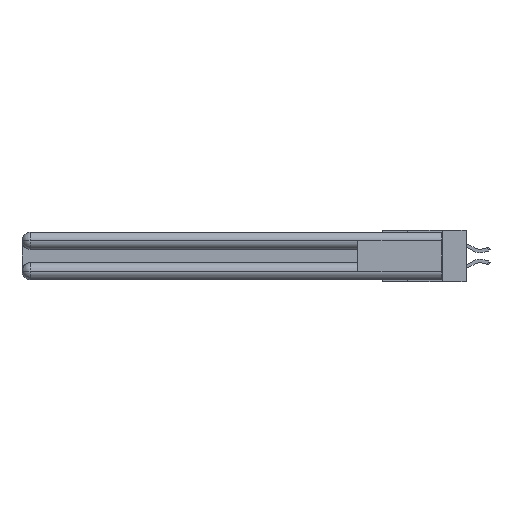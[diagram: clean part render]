
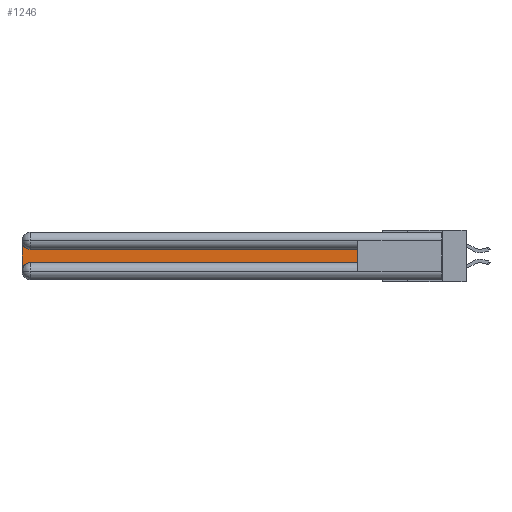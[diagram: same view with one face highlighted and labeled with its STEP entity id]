
A CAD part, left-side view. The second image highlights one B-rep face of the part: STEP entity #1246.
In plain terms, the highlighted planar face has unit normal (-1, 0, 0).
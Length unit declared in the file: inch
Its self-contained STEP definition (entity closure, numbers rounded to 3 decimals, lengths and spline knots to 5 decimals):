
#1246 = ADVANCED_FACE ( 'NONE', ( #10459 ), #15088, .F. ) ;
#3960 = AXIS2_PLACEMENT_3D ( 'NONE', #13023, #15390, #19690 ) ;
#4750 = CARTESIAN_POINT ( 'NONE',  ( 0.075, 3., -0.0625 ) ) ;
#5403 = DIRECTION ( 'NONE',  ( 0., 1., 0. ) ) ;
#7735 = DIRECTION ( 'NONE',  ( 1., 0., 0. ) ) ;
#7924 = AXIS2_PLACEMENT_3D ( 'NONE', #18759, #21262, #21171 ) ;
#8224 = ORIENTED_EDGE ( 'NONE', *, *, #29377, .T. ) ;
#9787 = DIRECTION ( 'NONE',  ( 0., 0., 1. ) ) ;
#9910 = CARTESIAN_POINT ( 'NONE',  ( 0.075, 3., -0.2175 ) ) ;
#9978 = VERTEX_POINT ( 'NONE', #19123 ) ;
#10459 = FACE_OUTER_BOUND ( 'NONE', #13842, .T. ) ;
#11279 = EDGE_CURVE ( 'NONE', #16786, #24887, #27911, .T. ) ;
#12070 = CARTESIAN_POINT ( 'NONE',  ( 0.075, 2.94, -0.2175 ) ) ;
#12254 = EDGE_CURVE ( 'NONE', #24251, #9978, #27850, .T. ) ;
#12385 = DIRECTION ( 'NONE',  ( 0., 0., -1. ) ) ;
#12804 = VERTEX_POINT ( 'NONE', #12070 ) ;
#13015 = EDGE_CURVE ( 'NONE', #24887, #21343, #20243, .T. ) ;
#13023 = CARTESIAN_POINT ( 'NONE',  ( 0.075, 3., -0.1225 ) ) ;
#13842 = EDGE_LOOP ( 'NONE', ( #17385, #18040, #17918, #13996, #8224, #17366 ) ) ;
#13996 = ORIENTED_EDGE ( 'NONE', *, *, #31014, .T. ) ;
#15088 = PLANE ( 'NONE',  #3960 ) ;
#15390 = DIRECTION ( 'NONE',  ( 1., 0., 0. ) ) ;
#16305 = LINE ( 'NONE', #22502, #21920 ) ;
#16652 = CARTESIAN_POINT ( 'NONE',  ( 0.075, 0.6, -0.1225 ) ) ;
#16786 = VERTEX_POINT ( 'NONE', #24002 ) ;
#17366 = ORIENTED_EDGE ( 'NONE', *, *, #11279, .T. ) ;
#17385 = ORIENTED_EDGE ( 'NONE', *, *, #13015, .T. ) ;
#17850 = CIRCLE ( 'NONE', #27565, 0.06 ) ;
#17918 = ORIENTED_EDGE ( 'NONE', *, *, #12254, .T. ) ;
#18040 = ORIENTED_EDGE ( 'NONE', *, *, #29230, .T. ) ;
#18412 = VECTOR ( 'NONE', #5403, 39.37008 ) ;
#18759 = CARTESIAN_POINT ( 'NONE',  ( 0.075, 2.94, -0.2775 ) ) ;
#19123 = CARTESIAN_POINT ( 'NONE',  ( 0.075, 3., -0.2775 ) ) ;
#19690 = DIRECTION ( 'NONE',  ( 0., 0., -1. ) ) ;
#20243 = LINE ( 'NONE', #29111, #18412 ) ;
#21171 = DIRECTION ( 'NONE',  ( 0., 0., -1. ) ) ;
#21262 = DIRECTION ( 'NONE',  ( 1., 0., 0. ) ) ;
#21343 = VERTEX_POINT ( 'NONE', #24619 ) ;
#21473 = VECTOR ( 'NONE', #26629, 39.37008 ) ;
#21920 = VECTOR ( 'NONE', #22296, 39.37008 ) ;
#22296 = DIRECTION ( 'NONE',  ( 0., -1., 0. ) ) ;
#22502 = CARTESIAN_POINT ( 'NONE',  ( 0.075, 0.6, -0.2175 ) ) ;
#24002 = CARTESIAN_POINT ( 'NONE',  ( 0.075, 0.6, -0.2175 ) ) ;
#24136 = CARTESIAN_POINT ( 'NONE',  ( 0.075, 0.6, -0.2175 ) ) ;
#24251 = VERTEX_POINT ( 'NONE', #4750 ) ;
#24619 = CARTESIAN_POINT ( 'NONE',  ( 0.075, 2.94, -0.1225 ) ) ;
#24887 = VERTEX_POINT ( 'NONE', #16652 ) ;
#26629 = DIRECTION ( 'NONE',  ( 0., 0., -1. ) ) ;
#26810 = CARTESIAN_POINT ( 'NONE',  ( 0.075, 2.94, -0.0625 ) ) ;
#27098 = CIRCLE ( 'NONE', #7924, 0.06 ) ;
#27565 = AXIS2_PLACEMENT_3D ( 'NONE', #26810, #7735, #12385 ) ;
#27850 = LINE ( 'NONE', #9910, #21473 ) ;
#27911 = LINE ( 'NONE', #24136, #30909 ) ;
#29111 = CARTESIAN_POINT ( 'NONE',  ( 0.075, 0.6, -0.1225 ) ) ;
#29230 = EDGE_CURVE ( 'NONE', #21343, #24251, #17850, .T. ) ;
#29377 = EDGE_CURVE ( 'NONE', #12804, #16786, #16305, .T. ) ;
#30909 = VECTOR ( 'NONE', #9787, 39.37008 ) ;
#31014 = EDGE_CURVE ( 'NONE', #9978, #12804, #27098, .T. ) ;
